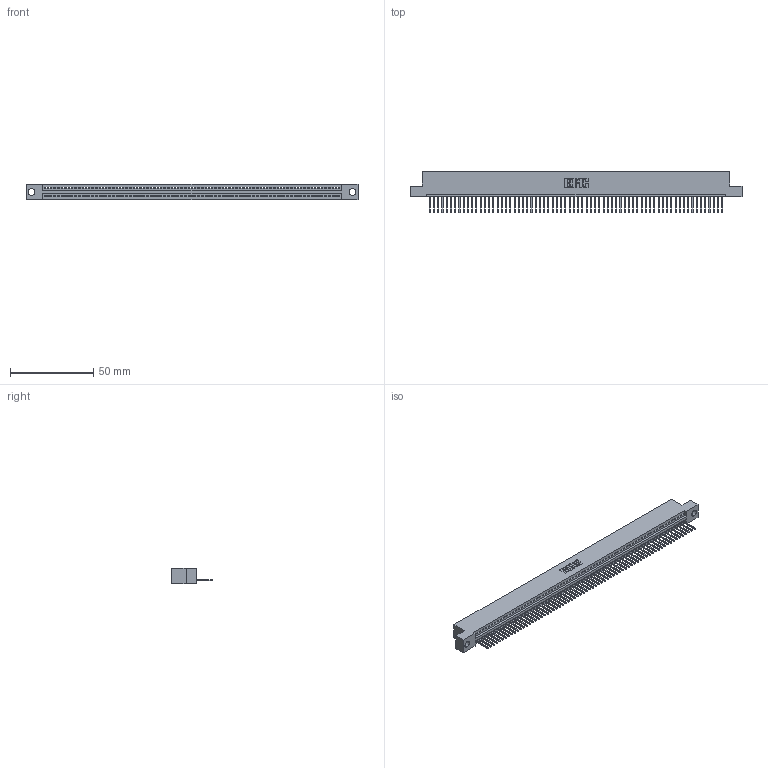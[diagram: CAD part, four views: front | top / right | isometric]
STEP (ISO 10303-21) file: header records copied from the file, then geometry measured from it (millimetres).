
FILE_DESCRIPTION (( 'STEP AP203' ), '1' );
FILE_NAME ('395-070-523-104.STEP', '2021-05-31T22:19:10', ( '' ), ( '' ), 'SwSTEP 2.0', 'SolidWorks 2020', '' );
FILE_SCHEMA (( 'CONFIG_CONTROL_DESIGN' ));
Length unit declared in the file: inch
Products named in the file (3): 345-292-001_345-293-123; 395-070-523-104; 345 Part_Flush Mounting Lugs - 0.156 Dia-TI
Assembly tree (71 placements, depth 2):
  395-070-523-104
    345 Part_Flush Mounting Lugs - 0.156 Dia-TI
    345-292-001_345-293-123  x70
Bounding box: 199.01 x 24.82 x 9.4 mm (x, y, z)
Volume: 18998.4 mm3; surface area: 25546.5 mm2
Topology: 71 solids, 71 shells, 4200 faces, 12697 edges, 8370 vertices
Faces by surface type: plane 2894, cylinder 1306
Entity records: 49351 total; most frequent: ORIENTED_EDGE 8558, CARTESIAN_POINT 8556, DIRECTION 7431, EDGE_CURVE 4279, VECTOR 3867, LINE 3867, VERTEX_POINT 2850, AXIS2_PLACEMENT_3D 1782
